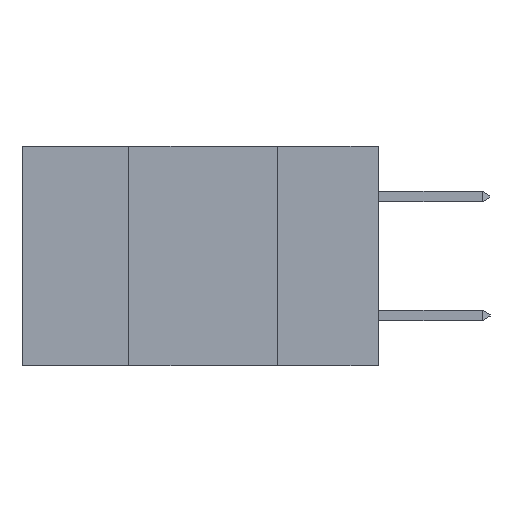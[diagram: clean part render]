
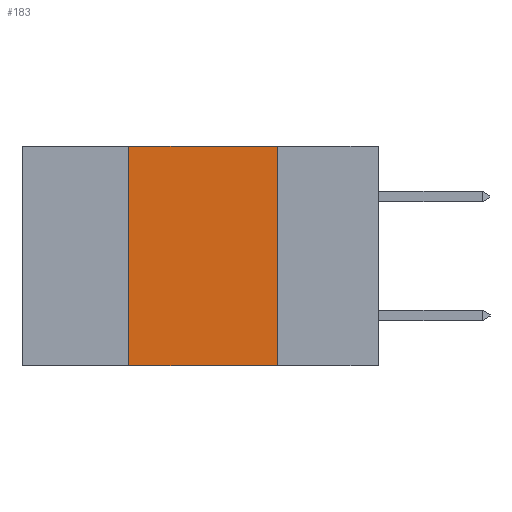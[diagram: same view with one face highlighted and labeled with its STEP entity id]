
A CAD part, left-side view. The second image highlights one B-rep face of the part: STEP entity #183.
In plain terms, the highlighted planar face has unit normal (-1, 0, 0).
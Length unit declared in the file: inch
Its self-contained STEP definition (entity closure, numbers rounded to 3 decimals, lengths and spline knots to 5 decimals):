
#28 = EDGE_CURVE ( 'NONE', #3559, #10150, #8048, .T. ) ;
#183 = ADVANCED_FACE ( 'NONE', ( #6741 ), #5624, .F. ) ;
#611 = CARTESIAN_POINT ( 'NONE',  ( 0., 0.6, -0.37 ) ) ;
#798 = EDGE_CURVE ( 'NONE', #3559, #1177, #5150, .T. ) ;
#827 = DIRECTION ( 'NONE',  ( 0., 0., -1. ) ) ;
#938 = VECTOR ( 'NONE', #11681, 39.37008 ) ;
#1177 = VERTEX_POINT ( 'NONE', #3163 ) ;
#1318 = CARTESIAN_POINT ( 'NONE',  ( 0., 0.42, -0.37 ) ) ;
#2203 = VERTEX_POINT ( 'NONE', #9065 ) ;
#2394 = EDGE_LOOP ( 'NONE', ( #8214, #12471, #13234, #7034 ) ) ;
#2562 = VECTOR ( 'NONE', #13299, 39.37008 ) ;
#3163 = CARTESIAN_POINT ( 'NONE',  ( 0., 0.42, 0. ) ) ;
#3559 = VERTEX_POINT ( 'NONE', #1318 ) ;
#3730 = CARTESIAN_POINT ( 'NONE',  ( 0., 0.6, 0. ) ) ;
#3945 = LINE ( 'NONE', #4544, #938 ) ;
#3950 = DIRECTION ( 'NONE',  ( 0., -1., 0. ) ) ;
#4544 = CARTESIAN_POINT ( 'NONE',  ( 0., 0.17, -0.37 ) ) ;
#5150 = LINE ( 'NONE', #10249, #2562 ) ;
#5320 = VECTOR ( 'NONE', #3950, 39.37008 ) ;
#5387 = DIRECTION ( 'NONE',  ( 1., 0., 0. ) ) ;
#5439 = CARTESIAN_POINT ( 'NONE',  ( 0., 0.17, -0.37 ) ) ;
#5624 = PLANE ( 'NONE',  #9778 ) ;
#6741 = FACE_OUTER_BOUND ( 'NONE', #2394, .T. ) ;
#6828 = VECTOR ( 'NONE', #10110, 39.37008 ) ;
#7034 = ORIENTED_EDGE ( 'NONE', *, *, #28, .T. ) ;
#7483 = LINE ( 'NONE', #9081, #6828 ) ;
#8048 = LINE ( 'NONE', #611, #5320 ) ;
#8214 = ORIENTED_EDGE ( 'NONE', *, *, #9025, .F. ) ;
#9025 = EDGE_CURVE ( 'NONE', #2203, #10150, #3945, .T. ) ;
#9065 = CARTESIAN_POINT ( 'NONE',  ( 0., 0.17, 0. ) ) ;
#9081 = CARTESIAN_POINT ( 'NONE',  ( 0., 0.6, 0. ) ) ;
#9778 = AXIS2_PLACEMENT_3D ( 'NONE', #3730, #5387, #827 ) ;
#10110 = DIRECTION ( 'NONE',  ( 0., -1., 0. ) ) ;
#10150 = VERTEX_POINT ( 'NONE', #5439 ) ;
#10249 = CARTESIAN_POINT ( 'NONE',  ( 0., 0.42, -0.37 ) ) ;
#11180 = EDGE_CURVE ( 'NONE', #1177, #2203, #7483, .T. ) ;
#11681 = DIRECTION ( 'NONE',  ( 0., 0., -1. ) ) ;
#12471 = ORIENTED_EDGE ( 'NONE', *, *, #11180, .F. ) ;
#13234 = ORIENTED_EDGE ( 'NONE', *, *, #798, .F. ) ;
#13299 = DIRECTION ( 'NONE',  ( 0., 0., 1. ) ) ;
